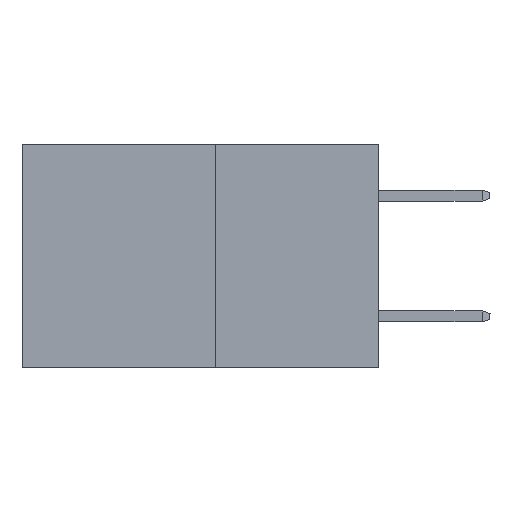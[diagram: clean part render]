
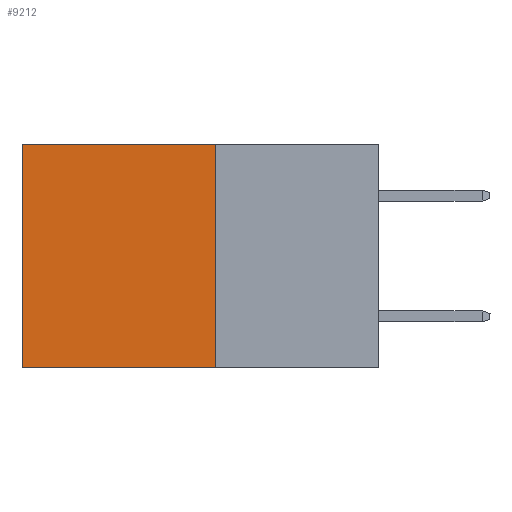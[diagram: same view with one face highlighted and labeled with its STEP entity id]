
A CAD part, left-side view. The second image highlights one B-rep face of the part: STEP entity #9212.
In plain terms, the highlighted planar face has unit normal (-1, 0, 0).
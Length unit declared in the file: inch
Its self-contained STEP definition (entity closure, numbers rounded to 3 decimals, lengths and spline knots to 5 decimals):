
#89 = ORIENTED_EDGE ( 'NONE', *, *, #223, .T. ) ;
#223 = EDGE_CURVE ( 'NONE', #7287, #6948, #1479, .T. ) ;
#502 = EDGE_CURVE ( 'NONE', #4591, #7287, #8138, .T. ) ;
#963 = ORIENTED_EDGE ( 'NONE', *, *, #2184, .F. ) ;
#1479 = LINE ( 'NONE', #5119, #7594 ) ;
#1663 = EDGE_CURVE ( 'NONE', #8620, #6948, #7987, .T. ) ;
#2184 = EDGE_CURVE ( 'NONE', #4591, #8620, #5710, .T. ) ;
#3021 = CARTESIAN_POINT ( 'NONE',  ( 0.277, 0.27, -0.37 ) ) ;
#3150 = VECTOR ( 'NONE', #10074, 39.37008 ) ;
#3163 = ORIENTED_EDGE ( 'NONE', *, *, #502, .T. ) ;
#3982 = CARTESIAN_POINT ( 'NONE',  ( 0.277, 0.27, 0. ) ) ;
#4585 = DIRECTION ( 'NONE',  ( 0., 1., 0. ) ) ;
#4591 = VERTEX_POINT ( 'NONE', #5581 ) ;
#5046 = DIRECTION ( 'NONE',  ( 1., 0., 0. ) ) ;
#5119 = CARTESIAN_POINT ( 'NONE',  ( 0.277, 0.59, -0.37 ) ) ;
#5581 = CARTESIAN_POINT ( 'NONE',  ( 0.277, 0.27, 0. ) ) ;
#5710 = LINE ( 'NONE', #9222, #3150 ) ;
#6253 = ORIENTED_EDGE ( 'NONE', *, *, #1663, .F. ) ;
#6465 = DIRECTION ( 'NONE',  ( 0., 0., -1. ) ) ;
#6948 = VERTEX_POINT ( 'NONE', #10357 ) ;
#7287 = VERTEX_POINT ( 'NONE', #8482 ) ;
#7594 = VECTOR ( 'NONE', #6465, 39.37008 ) ;
#7703 = FACE_OUTER_BOUND ( 'NONE', #9830, .T. ) ;
#7766 = VECTOR ( 'NONE', #8877, 39.37008 ) ;
#7987 = LINE ( 'NONE', #8831, #7766 ) ;
#8138 = LINE ( 'NONE', #3982, #10209 ) ;
#8482 = CARTESIAN_POINT ( 'NONE',  ( 0.277, 0.59, 0. ) ) ;
#8574 = AXIS2_PLACEMENT_3D ( 'NONE', #9371, #5046, #10062 ) ;
#8620 = VERTEX_POINT ( 'NONE', #3021 ) ;
#8645 = PLANE ( 'NONE',  #8574 ) ;
#8831 = CARTESIAN_POINT ( 'NONE',  ( 0.277, 0.27, -0.37 ) ) ;
#8877 = DIRECTION ( 'NONE',  ( 0., 1., 0. ) ) ;
#9212 = ADVANCED_FACE ( 'NONE', ( #7703 ), #8645, .F. ) ;
#9222 = CARTESIAN_POINT ( 'NONE',  ( 0.277, 0.27, -0.37 ) ) ;
#9371 = CARTESIAN_POINT ( 'NONE',  ( 0.277, 0.27, -0.37 ) ) ;
#9830 = EDGE_LOOP ( 'NONE', ( #89, #6253, #963, #3163 ) ) ;
#10062 = DIRECTION ( 'NONE',  ( 0., 0., -1. ) ) ;
#10074 = DIRECTION ( 'NONE',  ( 0., 0., -1. ) ) ;
#10209 = VECTOR ( 'NONE', #4585, 39.37008 ) ;
#10357 = CARTESIAN_POINT ( 'NONE',  ( 0.277, 0.59, -0.37 ) ) ;
